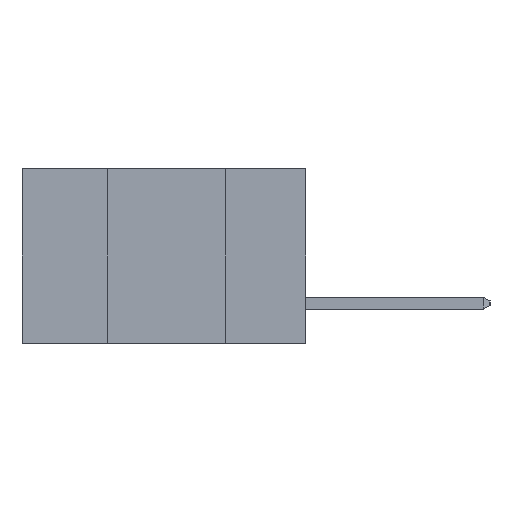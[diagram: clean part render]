
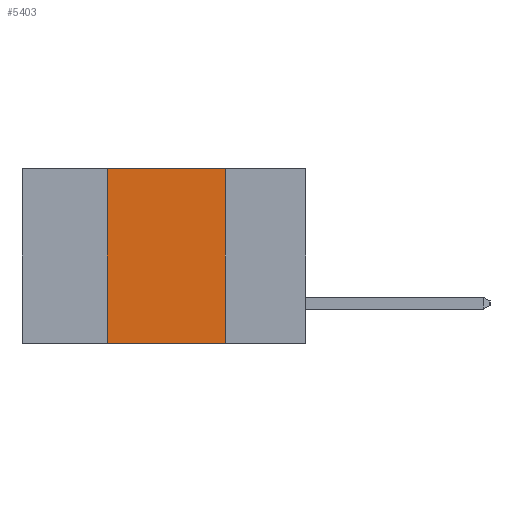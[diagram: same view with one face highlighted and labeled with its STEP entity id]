
A CAD part, left-side view. The second image highlights one B-rep face of the part: STEP entity #5403.
In plain terms, the highlighted planar face has unit normal (-1, 0, 0).
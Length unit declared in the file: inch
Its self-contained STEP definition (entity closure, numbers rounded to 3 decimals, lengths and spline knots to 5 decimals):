
#328 = FACE_OUTER_BOUND ( 'NONE', #12415, .T. ) ;
#614 = CARTESIAN_POINT ( 'NONE',  ( 0., 0.17, -0.37 ) ) ;
#1023 = DIRECTION ( 'NONE',  ( 0., 0., 1. ) ) ;
#1042 = CARTESIAN_POINT ( 'NONE',  ( 0., 0.6, 0. ) ) ;
#1053 = ORIENTED_EDGE ( 'NONE', *, *, #8015, .T. ) ;
#1364 = EDGE_CURVE ( 'NONE', #13054, #13276, #11537, .T. ) ;
#1550 = VERTEX_POINT ( 'NONE', #614 ) ;
#1581 = VECTOR ( 'NONE', #1991, 39.37008 ) ;
#1669 = CARTESIAN_POINT ( 'NONE',  ( 0., 0.42, 0. ) ) ;
#1991 = DIRECTION ( 'NONE',  ( 0., -1., 0. ) ) ;
#3535 = ORIENTED_EDGE ( 'NONE', *, *, #4031, .F. ) ;
#3873 = DIRECTION ( 'NONE',  ( 1., 0., 0. ) ) ;
#3907 = PLANE ( 'NONE',  #8476 ) ;
#4031 = EDGE_CURVE ( 'NONE', #10000, #13054, #8115, .T. ) ;
#5403 = ADVANCED_FACE ( 'NONE', ( #328 ), #3907, .F. ) ;
#5433 = DIRECTION ( 'NONE',  ( 0., -1., 0. ) ) ;
#6053 = DIRECTION ( 'NONE',  ( 0., 0., -1. ) ) ;
#6575 = CARTESIAN_POINT ( 'NONE',  ( 0., 0.42, 0. ) ) ;
#8015 = EDGE_CURVE ( 'NONE', #10000, #1550, #8933, .T. ) ;
#8115 = LINE ( 'NONE', #6575, #10905 ) ;
#8202 = VECTOR ( 'NONE', #5433, 39.37008 ) ;
#8476 = AXIS2_PLACEMENT_3D ( 'NONE', #8992, #3873, #6053 ) ;
#8867 = CARTESIAN_POINT ( 'NONE',  ( 0., 0.42, -0.37 ) ) ;
#8933 = LINE ( 'NONE', #10171, #8202 ) ;
#8992 = CARTESIAN_POINT ( 'NONE',  ( 0., 0.6, 0. ) ) ;
#9324 = CARTESIAN_POINT ( 'NONE',  ( 0., 0.17, 0. ) ) ;
#10000 = VERTEX_POINT ( 'NONE', #8867 ) ;
#10171 = CARTESIAN_POINT ( 'NONE',  ( 0., 0.6, -0.37 ) ) ;
#10443 = ORIENTED_EDGE ( 'NONE', *, *, #15081, .F. ) ;
#10554 = DIRECTION ( 'NONE',  ( 0., 0., -1. ) ) ;
#10905 = VECTOR ( 'NONE', #1023, 39.37008 ) ;
#11537 = LINE ( 'NONE', #1042, #1581 ) ;
#11730 = CARTESIAN_POINT ( 'NONE',  ( 0., 0.17, 0. ) ) ;
#12415 = EDGE_LOOP ( 'NONE', ( #10443, #14248, #3535, #1053 ) ) ;
#13054 = VERTEX_POINT ( 'NONE', #1669 ) ;
#13276 = VERTEX_POINT ( 'NONE', #11730 ) ;
#14248 = ORIENTED_EDGE ( 'NONE', *, *, #1364, .F. ) ;
#14663 = VECTOR ( 'NONE', #10554, 39.37008 ) ;
#15008 = LINE ( 'NONE', #9324, #14663 ) ;
#15081 = EDGE_CURVE ( 'NONE', #13276, #1550, #15008, .T. ) ;
